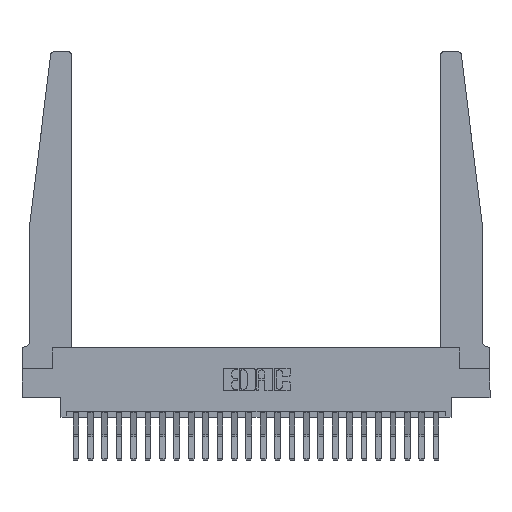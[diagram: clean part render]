
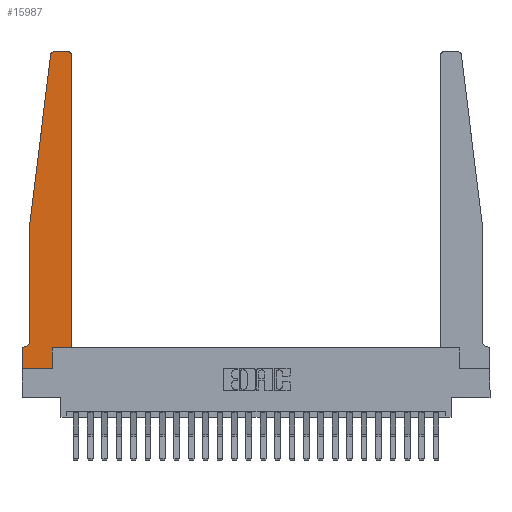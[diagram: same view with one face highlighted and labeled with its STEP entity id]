
A CAD part, top view. The second image highlights one B-rep face of the part: STEP entity #15987.
In plain terms, the highlighted planar face has unit normal (0, 0, 1).
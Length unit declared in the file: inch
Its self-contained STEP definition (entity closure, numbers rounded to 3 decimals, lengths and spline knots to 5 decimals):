
#552 = VERTEX_POINT ( 'NONE', #9131 ) ;
#591 = VERTEX_POINT ( 'NONE', #8590 ) ;
#607 = CARTESIAN_POINT ( 'NONE',  ( 0., 0.1875, 0.37 ) ) ;
#747 = CARTESIAN_POINT ( 'NONE',  ( 0.2605, 0.18, 0.37 ) ) ;
#760 = VERTEX_POINT ( 'NONE', #17026 ) ;
#1184 = LINE ( 'NONE', #18500, #10055 ) ;
#1461 = CARTESIAN_POINT ( 'NONE',  ( 0.2605, 0., 0.37 ) ) ;
#1512 = ORIENTED_EDGE ( 'NONE', *, *, #19683, .T. ) ;
#1607 = DIRECTION ( 'NONE',  ( -0.122, -0.992, 0. ) ) ;
#1647 = FACE_OUTER_BOUND ( 'NONE', #22921, .T. ) ;
#1686 = LINE ( 'NONE', #21976, #21048 ) ;
#2113 = CARTESIAN_POINT ( 'NONE',  ( 0.395, 2.75, 0.37 ) ) ;
#2303 = CARTESIAN_POINT ( 'NONE',  ( 0.015, 0.2375, 0.37 ) ) ;
#2409 = VECTOR ( 'NONE', #17453, 39.37008 ) ;
#2483 = DIRECTION ( 'NONE',  ( 1., 0., 0. ) ) ;
#2615 = VERTEX_POINT ( 'NONE', #11409 ) ;
#2757 = CARTESIAN_POINT ( 'NONE',  ( 0., 0., 0.37 ) ) ;
#2946 = CARTESIAN_POINT ( 'NONE',  ( 0.2605, 0.18, 0.37 ) ) ;
#3335 = DIRECTION ( 'NONE',  ( 0., 0., 1. ) ) ;
#3676 = EDGE_CURVE ( 'NONE', #14515, #15397, #21610, .T. ) ;
#3827 = EDGE_CURVE ( 'NONE', #5684, #7507, #14345, .T. ) ;
#4214 = DIRECTION ( 'NONE',  ( -1., 0., 0. ) ) ;
#4548 = ORIENTED_EDGE ( 'NONE', *, *, #13738, .T. ) ;
#4599 = CIRCLE ( 'NONE', #10912, 0.03 ) ;
#4852 = LINE ( 'NONE', #7177, #24036 ) ;
#4867 = ORIENTED_EDGE ( 'NONE', *, *, #6314, .T. ) ;
#5098 = DIRECTION ( 'NONE',  ( 1., 0., 0. ) ) ;
#5327 = DIRECTION ( 'NONE',  ( 0., 1., 0. ) ) ;
#5424 = CARTESIAN_POINT ( 'NONE',  ( 0.27653, 2.72, 0.37 ) ) ;
#5684 = VERTEX_POINT ( 'NONE', #1461 ) ;
#6123 = CARTESIAN_POINT ( 'NONE',  ( 0.065, 1.25, 0.37 ) ) ;
#6216 = PLANE ( 'NONE',  #9727 ) ;
#6263 = CARTESIAN_POINT ( 'NONE',  ( 0.425, 0.18, 0.37 ) ) ;
#6314 = EDGE_CURVE ( 'NONE', #552, #9355, #4599, .T. ) ;
#7177 = CARTESIAN_POINT ( 'NONE',  ( 0.425, 0.18, 0.37 ) ) ;
#7349 = DIRECTION ( 'NONE',  ( 1., 0., 0. ) ) ;
#7415 = CARTESIAN_POINT ( 'NONE',  ( 0.425, 0.18, 0.37 ) ) ;
#7432 = ORIENTED_EDGE ( 'NONE', *, *, #8723, .T. ) ;
#7507 = VERTEX_POINT ( 'NONE', #2946 ) ;
#7711 = ORIENTED_EDGE ( 'NONE', *, *, #14995, .T. ) ;
#8017 = DIRECTION ( 'NONE',  ( 0., -1., 0. ) ) ;
#8063 = CARTESIAN_POINT ( 'NONE',  ( 0.015, 0.1875, 0.37 ) ) ;
#8144 = EDGE_CURVE ( 'NONE', #23710, #22811, #19821, .T. ) ;
#8590 = CARTESIAN_POINT ( 'NONE',  ( 0.27653, 2.75, 0.37 ) ) ;
#8723 = EDGE_CURVE ( 'NONE', #760, #14515, #17466, .T. ) ;
#8734 = ORIENTED_EDGE ( 'NONE', *, *, #8144, .T. ) ;
#9131 = CARTESIAN_POINT ( 'NONE',  ( 0.425, 2.72, 0.37 ) ) ;
#9355 = VERTEX_POINT ( 'NONE', #2113 ) ;
#9727 = AXIS2_PLACEMENT_3D ( 'NONE', #607, #13729, #2483 ) ;
#9840 = LINE ( 'NONE', #22122, #19736 ) ;
#10055 = VECTOR ( 'NONE', #1607, 39.37008 ) ;
#10912 = AXIS2_PLACEMENT_3D ( 'NONE', #14568, #3335, #16453 ) ;
#11081 = EDGE_CURVE ( 'NONE', #591, #2615, #18866, .T. ) ;
#11409 = CARTESIAN_POINT ( 'NONE',  ( 0.24675, 2.72367, 0.37 ) ) ;
#11418 = EDGE_CURVE ( 'NONE', #7507, #20131, #12988, .T. ) ;
#11462 = ORIENTED_EDGE ( 'NONE', *, *, #11418, .T. ) ;
#11635 = CARTESIAN_POINT ( 'NONE',  ( 0., 0., 0.37 ) ) ;
#12502 = ORIENTED_EDGE ( 'NONE', *, *, #17938, .T. ) ;
#12988 = LINE ( 'NONE', #6263, #2409 ) ;
#13729 = DIRECTION ( 'NONE',  ( 0., 0., 1. ) ) ;
#13738 = EDGE_CURVE ( 'NONE', #9355, #591, #1686, .T. ) ;
#13986 = ORIENTED_EDGE ( 'NONE', *, *, #3827, .T. ) ;
#14345 = LINE ( 'NONE', #747, #20248 ) ;
#14439 = CARTESIAN_POINT ( 'NONE',  ( 0., 0., 0.37 ) ) ;
#14515 = VERTEX_POINT ( 'NONE', #22473 ) ;
#14568 = CARTESIAN_POINT ( 'NONE',  ( 0.395, 2.72, 0.37 ) ) ;
#14995 = EDGE_CURVE ( 'NONE', #22811, #5684, #16929, .T. ) ;
#15397 = VERTEX_POINT ( 'NONE', #8063 ) ;
#15440 = DIRECTION ( 'NONE',  ( 0., 0., -1. ) ) ;
#15755 = VECTOR ( 'NONE', #5098, 39.37008 ) ;
#15757 = DIRECTION ( 'NONE',  ( 0., 1., 0. ) ) ;
#15887 = DIRECTION ( 'NONE',  ( 0., -1., 0. ) ) ;
#15987 = ADVANCED_FACE ( 'NONE', ( #1647 ), #6216, .T. ) ;
#16398 = DIRECTION ( 'NONE',  ( -1., 0., 0. ) ) ;
#16453 = DIRECTION ( 'NONE',  ( 1., 0., 0. ) ) ;
#16874 = VECTOR ( 'NONE', #8017, 39.37008 ) ;
#16929 = LINE ( 'NONE', #14439, #15755 ) ;
#17010 = EDGE_CURVE ( 'NONE', #20131, #552, #4852, .T. ) ;
#17026 = CARTESIAN_POINT ( 'NONE',  ( 0.065, 1.25, 0.37 ) ) ;
#17453 = DIRECTION ( 'NONE',  ( 1., 0., 0. ) ) ;
#17466 = LINE ( 'NONE', #6123, #16874 ) ;
#17938 = EDGE_CURVE ( 'NONE', #15397, #23710, #9840, .T. ) ;
#18030 = ORIENTED_EDGE ( 'NONE', *, *, #11081, .T. ) ;
#18047 = AXIS2_PLACEMENT_3D ( 'NONE', #2303, #15440, #4214 ) ;
#18500 = CARTESIAN_POINT ( 'NONE',  ( 0.065, 1.25, 0.37 ) ) ;
#18519 = DIRECTION ( 'NONE',  ( 0., 0., 1. ) ) ;
#18866 = CIRCLE ( 'NONE', #20407, 0.03 ) ;
#19252 = VECTOR ( 'NONE', #15887, 39.37008 ) ;
#19683 = EDGE_CURVE ( 'NONE', #2615, #760, #1184, .T. ) ;
#19736 = VECTOR ( 'NONE', #23929, 39.37008 ) ;
#19821 = LINE ( 'NONE', #2757, #19252 ) ;
#20131 = VERTEX_POINT ( 'NONE', #7415 ) ;
#20248 = VECTOR ( 'NONE', #15757, 39.37008 ) ;
#20401 = CARTESIAN_POINT ( 'NONE',  ( 0., 0.1875, 0.37 ) ) ;
#20407 = AXIS2_PLACEMENT_3D ( 'NONE', #5424, #18519, #7349 ) ;
#21048 = VECTOR ( 'NONE', #16398, 39.37008 ) ;
#21402 = ORIENTED_EDGE ( 'NONE', *, *, #17010, .T. ) ;
#21610 = CIRCLE ( 'NONE', #18047, 0.05 ) ;
#21976 = CARTESIAN_POINT ( 'NONE',  ( 0.25, 2.75, 0.37 ) ) ;
#22122 = CARTESIAN_POINT ( 'NONE',  ( 0.065, 0.1875, 0.37 ) ) ;
#22473 = CARTESIAN_POINT ( 'NONE',  ( 0.065, 0.2375, 0.37 ) ) ;
#22702 = ORIENTED_EDGE ( 'NONE', *, *, #3676, .T. ) ;
#22811 = VERTEX_POINT ( 'NONE', #11635 ) ;
#22921 = EDGE_LOOP ( 'NONE', ( #4548, #18030, #1512, #7432, #22702, #12502, #8734, #7711, #13986, #11462, #21402, #4867 ) ) ;
#23710 = VERTEX_POINT ( 'NONE', #20401 ) ;
#23929 = DIRECTION ( 'NONE',  ( -1., 0., 0. ) ) ;
#24036 = VECTOR ( 'NONE', #5327, 39.37008 ) ;
